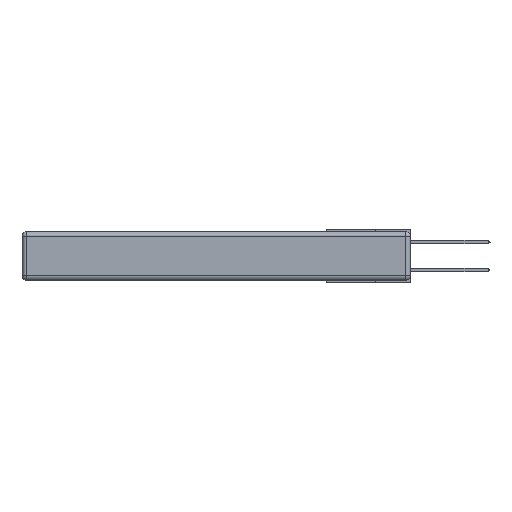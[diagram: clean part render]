
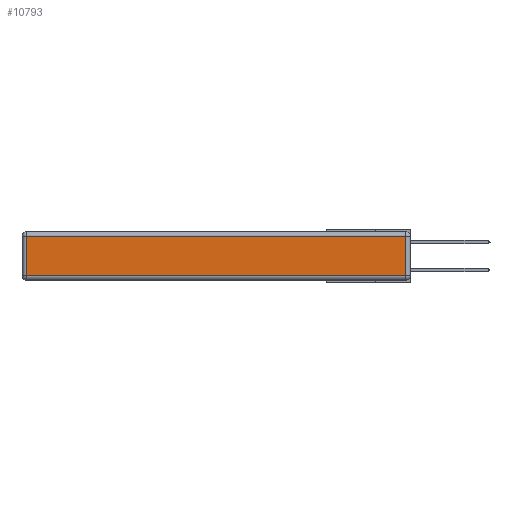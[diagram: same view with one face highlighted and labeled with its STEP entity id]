
A CAD part, left-side view. The second image highlights one B-rep face of the part: STEP entity #10793.
In plain terms, the highlighted planar face has unit normal (-1, 0, 0).
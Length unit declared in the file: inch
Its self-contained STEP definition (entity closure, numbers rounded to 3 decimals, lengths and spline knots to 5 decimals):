
#36 = VERTEX_POINT ( 'NONE', #11190 ) ;
#39 = LINE ( 'NONE', #14291, #8026 ) ;
#574 = DIRECTION ( 'NONE',  ( 0., -1., 0. ) ) ;
#798 = CARTESIAN_POINT ( 'NONE',  ( 0., 0., -0.343 ) ) ;
#4316 = DIRECTION ( 'NONE',  ( 0., 0., 1. ) ) ;
#4412 = CARTESIAN_POINT ( 'NONE',  ( 0., 0.03, -0.343 ) ) ;
#5489 = CARTESIAN_POINT ( 'NONE',  ( 0., 2.72, -0.03 ) ) ;
#5575 = VECTOR ( 'NONE', #10190, 39.37008 ) ;
#5873 = VERTEX_POINT ( 'NONE', #11923 ) ;
#6462 = LINE ( 'NONE', #9064, #9999 ) ;
#7450 = EDGE_CURVE ( 'NONE', #36, #5873, #14155, .T. ) ;
#7819 = CARTESIAN_POINT ( 'NONE',  ( 0., 2.72, -0.313 ) ) ;
#8026 = VECTOR ( 'NONE', #574, 39.37008 ) ;
#8438 = ORIENTED_EDGE ( 'NONE', *, *, #12675, .T. ) ;
#9049 = AXIS2_PLACEMENT_3D ( 'NONE', #798, #11061, #4316 ) ;
#9064 = CARTESIAN_POINT ( 'NONE',  ( 0., 2.72, -0.343 ) ) ;
#9415 = EDGE_LOOP ( 'NONE', ( #8438, #12334, #13716, #12452 ) ) ;
#9999 = VECTOR ( 'NONE', #10197, 39.37008 ) ;
#10093 = VECTOR ( 'NONE', #12335, 39.37008 ) ;
#10190 = DIRECTION ( 'NONE',  ( 0., 1., 0. ) ) ;
#10197 = DIRECTION ( 'NONE',  ( 0., 0., -1. ) ) ;
#10220 = VERTEX_POINT ( 'NONE', #5489 ) ;
#10793 = ADVANCED_FACE ( 'NONE', ( #12129 ), #10965, .T. ) ;
#10965 = PLANE ( 'NONE',  #9049 ) ;
#11001 = VERTEX_POINT ( 'NONE', #7819 ) ;
#11061 = DIRECTION ( 'NONE',  ( -1., 0., 0. ) ) ;
#11190 = CARTESIAN_POINT ( 'NONE',  ( 0., 0.03, -0.313 ) ) ;
#11250 = LINE ( 'NONE', #11279, #5575 ) ;
#11279 = CARTESIAN_POINT ( 'NONE',  ( 0., 2.75, -0.03 ) ) ;
#11923 = CARTESIAN_POINT ( 'NONE',  ( 0., 0.03, -0.03 ) ) ;
#12033 = EDGE_CURVE ( 'NONE', #5873, #10220, #11250, .T. ) ;
#12129 = FACE_OUTER_BOUND ( 'NONE', #9415, .T. ) ;
#12334 = ORIENTED_EDGE ( 'NONE', *, *, #7450, .T. ) ;
#12335 = DIRECTION ( 'NONE',  ( 0., 0., 1. ) ) ;
#12357 = EDGE_CURVE ( 'NONE', #10220, #11001, #6462, .T. ) ;
#12452 = ORIENTED_EDGE ( 'NONE', *, *, #12357, .T. ) ;
#12675 = EDGE_CURVE ( 'NONE', #11001, #36, #39, .T. ) ;
#13716 = ORIENTED_EDGE ( 'NONE', *, *, #12033, .T. ) ;
#14155 = LINE ( 'NONE', #4412, #10093 ) ;
#14291 = CARTESIAN_POINT ( 'NONE',  ( 0., 0., -0.313 ) ) ;
